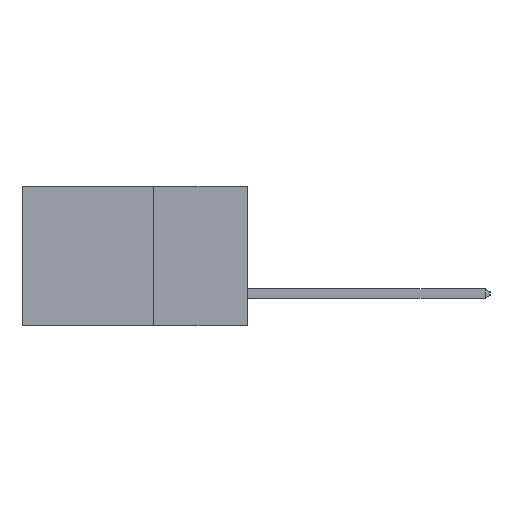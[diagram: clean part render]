
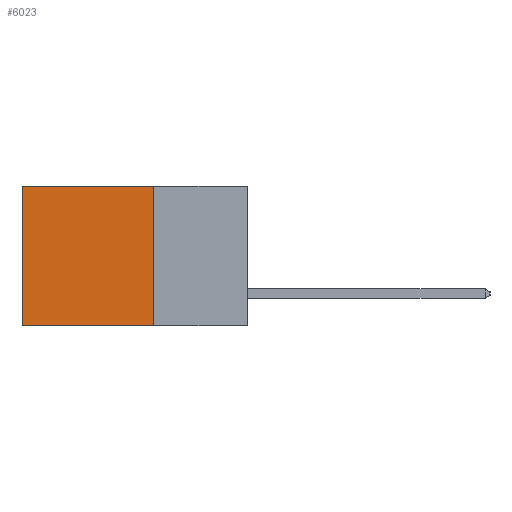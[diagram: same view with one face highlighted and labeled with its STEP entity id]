
A CAD part, left-side view. The second image highlights one B-rep face of the part: STEP entity #6023.
In plain terms, the highlighted planar face has unit normal (-1, 0, 0).
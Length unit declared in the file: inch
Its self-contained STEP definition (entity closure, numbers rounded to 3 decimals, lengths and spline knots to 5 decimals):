
#181 = EDGE_CURVE ( 'NONE', #12703, #4369, #11855, .T. ) ;
#922 = ORIENTED_EDGE ( 'NONE', *, *, #4583, .T. ) ;
#1584 = DIRECTION ( 'NONE',  ( 0., 1., 0. ) ) ;
#1591 = FACE_OUTER_BOUND ( 'NONE', #13657, .T. ) ;
#1593 = CARTESIAN_POINT ( 'NONE',  ( 0.298, 0.25, -0.37 ) ) ;
#1707 = EDGE_CURVE ( 'NONE', #4497, #2301, #3047, .T. ) ;
#1987 = CARTESIAN_POINT ( 'NONE',  ( 0.298, 0.6, 0. ) ) ;
#2189 = CARTESIAN_POINT ( 'NONE',  ( 0.298, 0.6, -0.37 ) ) ;
#2282 = LINE ( 'NONE', #10304, #10497 ) ;
#2301 = VERTEX_POINT ( 'NONE', #2189 ) ;
#2595 = CARTESIAN_POINT ( 'NONE',  ( 0.298, 0.25, 0. ) ) ;
#3047 = LINE ( 'NONE', #1593, #5538 ) ;
#3236 = EDGE_CURVE ( 'NONE', #12703, #4497, #2282, .T. ) ;
#3375 = CARTESIAN_POINT ( 'NONE',  ( 0.298, 0.25, -0.37 ) ) ;
#4369 = VERTEX_POINT ( 'NONE', #1987 ) ;
#4497 = VERTEX_POINT ( 'NONE', #3375 ) ;
#4583 = EDGE_CURVE ( 'NONE', #4369, #2301, #10301, .T. ) ;
#4660 = ORIENTED_EDGE ( 'NONE', *, *, #1707, .F. ) ;
#5416 = AXIS2_PLACEMENT_3D ( 'NONE', #6315, #13966, #7379 ) ;
#5538 = VECTOR ( 'NONE', #7882, 39.37008 ) ;
#5611 = CARTESIAN_POINT ( 'NONE',  ( 0.298, 0.25, 0. ) ) ;
#6023 = ADVANCED_FACE ( 'NONE', ( #1591 ), #12858, .F. ) ;
#6272 = DIRECTION ( 'NONE',  ( 0., 0., -1. ) ) ;
#6315 = CARTESIAN_POINT ( 'NONE',  ( 0.298, 0.25, 0. ) ) ;
#6753 = CARTESIAN_POINT ( 'NONE',  ( 0.298, 0.6, 0. ) ) ;
#7379 = DIRECTION ( 'NONE',  ( 0., 0., -1. ) ) ;
#7388 = VECTOR ( 'NONE', #6272, 39.37008 ) ;
#7882 = DIRECTION ( 'NONE',  ( 0., 1., 0. ) ) ;
#8417 = DIRECTION ( 'NONE',  ( 0., 0., -1. ) ) ;
#8830 = ORIENTED_EDGE ( 'NONE', *, *, #3236, .F. ) ;
#10301 = LINE ( 'NONE', #6753, #7388 ) ;
#10304 = CARTESIAN_POINT ( 'NONE',  ( 0.298, 0.25, 0. ) ) ;
#10497 = VECTOR ( 'NONE', #8417, 39.37008 ) ;
#11322 = ORIENTED_EDGE ( 'NONE', *, *, #181, .T. ) ;
#11855 = LINE ( 'NONE', #2595, #12224 ) ;
#12224 = VECTOR ( 'NONE', #1584, 39.37008 ) ;
#12703 = VERTEX_POINT ( 'NONE', #5611 ) ;
#12858 = PLANE ( 'NONE',  #5416 ) ;
#13657 = EDGE_LOOP ( 'NONE', ( #922, #4660, #8830, #11322 ) ) ;
#13966 = DIRECTION ( 'NONE',  ( 1., 0., 0. ) ) ;
